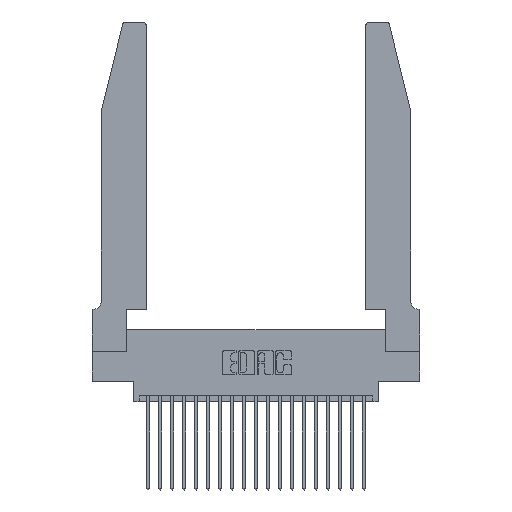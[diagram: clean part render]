
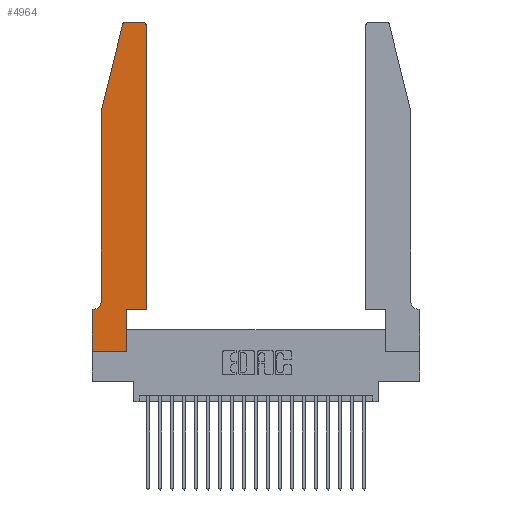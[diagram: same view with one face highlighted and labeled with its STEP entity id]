
A CAD part, top view. The second image highlights one B-rep face of the part: STEP entity #4964.
In plain terms, the highlighted planar face has unit normal (0, 0, 1).
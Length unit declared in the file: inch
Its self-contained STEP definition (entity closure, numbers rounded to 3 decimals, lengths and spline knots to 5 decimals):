
#15 = CARTESIAN_POINT ( 'NONE',  ( 0.0755, 2., 0.37 ) ) ;
#16 = LINE ( 'NONE', #1886, #22453 ) ;
#142 = CARTESIAN_POINT ( 'NONE',  ( 0.0755, 0.35, 0.37 ) ) ;
#749 = CARTESIAN_POINT ( 'NONE',  ( 0.0755, 2., 0.37 ) ) ;
#805 = DIRECTION ( 'NONE',  ( -0.239, -0.971, 0. ) ) ;
#913 = DIRECTION ( 'NONE',  ( 0., 0., 1. ) ) ;
#1130 = ORIENTED_EDGE ( 'NONE', *, *, #19484, .T. ) ;
#1185 = LINE ( 'NONE', #142, #15049 ) ;
#1429 = CIRCLE ( 'NONE', #18222, 0.03 ) ;
#1514 = EDGE_CURVE ( 'NONE', #3039, #11569, #1185, .T. ) ;
#1631 = DIRECTION ( 'NONE',  ( -1., 0., 0. ) ) ;
#1669 = DIRECTION ( 'NONE',  ( 1., 0., 0. ) ) ;
#1886 = CARTESIAN_POINT ( 'NONE',  ( 0.0755, 2., 0.37 ) ) ;
#1987 = ORIENTED_EDGE ( 'NONE', *, *, #20391, .T. ) ;
#2448 = LINE ( 'NONE', #13657, #20600 ) ;
#2665 = EDGE_CURVE ( 'NONE', #15918, #18695, #1429, .T. ) ;
#2792 = CARTESIAN_POINT ( 'NONE',  ( 0., 0.35, 0.37 ) ) ;
#3039 = VERTEX_POINT ( 'NONE', #20279 ) ;
#3133 = CARTESIAN_POINT ( 'NONE',  ( 0.0755, 0.42, 0.37 ) ) ;
#3229 = DIRECTION ( 'NONE',  ( 0., 0., -1. ) ) ;
#3417 = EDGE_CURVE ( 'NONE', #7662, #13350, #17607, .T. ) ;
#3521 = DIRECTION ( 'NONE',  ( 0., -1., 0. ) ) ;
#3588 = VERTEX_POINT ( 'NONE', #3133 ) ;
#3893 = VERTEX_POINT ( 'NONE', #21224 ) ;
#4565 = CARTESIAN_POINT ( 'NONE',  ( 0.4505, 0.35, 0.37 ) ) ;
#4650 = LINE ( 'NONE', #4565, #8903 ) ;
#4863 = AXIS2_PLACEMENT_3D ( 'NONE', #11895, #913, #13646 ) ;
#4964 = ADVANCED_FACE ( 'NONE', ( #22354 ), #22697, .T. ) ;
#5073 = LINE ( 'NONE', #21068, #18536 ) ;
#5251 = ORIENTED_EDGE ( 'NONE', *, *, #2665, .T. ) ;
#5435 = EDGE_CURVE ( 'NONE', #3588, #3039, #22332, .T. ) ;
#6041 = VERTEX_POINT ( 'NONE', #17377 ) ;
#7079 = ORIENTED_EDGE ( 'NONE', *, *, #11845, .T. ) ;
#7588 = VECTOR ( 'NONE', #21222, 39.37008 ) ;
#7662 = VERTEX_POINT ( 'NONE', #21555 ) ;
#7729 = ORIENTED_EDGE ( 'NONE', *, *, #5435, .T. ) ;
#8202 = VECTOR ( 'NONE', #3521, 39.37008 ) ;
#8570 = EDGE_CURVE ( 'NONE', #19285, #3893, #5073, .T. ) ;
#8903 = VECTOR ( 'NONE', #18604, 39.37008 ) ;
#9002 = CARTESIAN_POINT ( 'NONE',  ( 0., 0.35, 0.37 ) ) ;
#9226 = CARTESIAN_POINT ( 'NONE',  ( 0.2605, 2.75, 0.37 ) ) ;
#9789 = DIRECTION ( 'NONE',  ( 1., 0., 0. ) ) ;
#10373 = CARTESIAN_POINT ( 'NONE',  ( 0., 0., 0.37 ) ) ;
#11133 = CARTESIAN_POINT ( 'NONE',  ( 0.4505, 2.72, 0.37 ) ) ;
#11254 = EDGE_CURVE ( 'NONE', #13350, #3588, #16, .T. ) ;
#11338 = AXIS2_PLACEMENT_3D ( 'NONE', #13990, #3229, #15697 ) ;
#11569 = VERTEX_POINT ( 'NONE', #2792 ) ;
#11584 = CARTESIAN_POINT ( 'NONE',  ( 0., 0., 0.37 ) ) ;
#11598 = EDGE_CURVE ( 'NONE', #6041, #19285, #2448, .T. ) ;
#11786 = AXIS2_PLACEMENT_3D ( 'NONE', #9002, #12572, #1669 ) ;
#11804 = LINE ( 'NONE', #11584, #20334 ) ;
#11845 = EDGE_CURVE ( 'NONE', #11569, #17489, #20847, .T. ) ;
#11895 = CARTESIAN_POINT ( 'NONE',  ( 0.284, 2.72, 0.37 ) ) ;
#12526 = ORIENTED_EDGE ( 'NONE', *, *, #3417, .T. ) ;
#12572 = DIRECTION ( 'NONE',  ( 0., 0., 1. ) ) ;
#12629 = DIRECTION ( 'NONE',  ( 1., 0., 0. ) ) ;
#12766 = DIRECTION ( 'NONE',  ( 0., -1., 0. ) ) ;
#13350 = VERTEX_POINT ( 'NONE', #15 ) ;
#13523 = ORIENTED_EDGE ( 'NONE', *, *, #11598, .T. ) ;
#13646 = DIRECTION ( 'NONE',  ( 1., 0., 0. ) ) ;
#13657 = CARTESIAN_POINT ( 'NONE',  ( 0.2865, 0.35, 0.37 ) ) ;
#13990 = CARTESIAN_POINT ( 'NONE',  ( 0.0055, 0.42, 0.37 ) ) ;
#14261 = CARTESIAN_POINT ( 'NONE',  ( 0., 0., 0.37 ) ) ;
#14595 = ORIENTED_EDGE ( 'NONE', *, *, #15482, .T. ) ;
#15049 = VECTOR ( 'NONE', #1631, 39.37008 ) ;
#15482 = EDGE_CURVE ( 'NONE', #3893, #15918, #4650, .T. ) ;
#15697 = DIRECTION ( 'NONE',  ( -1., 0., 0. ) ) ;
#15918 = VERTEX_POINT ( 'NONE', #11133 ) ;
#16129 = ORIENTED_EDGE ( 'NONE', *, *, #16757, .T. ) ;
#16501 = EDGE_LOOP ( 'NONE', ( #1987, #16129, #12526, #22367, #7729, #19598, #7079, #1130, #13523, #19931, #14595, #5251 ) ) ;
#16757 = EDGE_CURVE ( 'NONE', #22017, #7662, #20162, .T. ) ;
#17085 = DIRECTION ( 'NONE',  ( 0., 1., 0. ) ) ;
#17116 = CARTESIAN_POINT ( 'NONE',  ( 0.284, 2.75, 0.37 ) ) ;
#17377 = CARTESIAN_POINT ( 'NONE',  ( 0.2865, 0., 0.37 ) ) ;
#17489 = VERTEX_POINT ( 'NONE', #10373 ) ;
#17607 = LINE ( 'NONE', #749, #20490 ) ;
#18222 = AXIS2_PLACEMENT_3D ( 'NONE', #19578, #19600, #19660 ) ;
#18536 = VECTOR ( 'NONE', #12629, 39.37008 ) ;
#18604 = DIRECTION ( 'NONE',  ( 0., 1., 0. ) ) ;
#18695 = VERTEX_POINT ( 'NONE', #19690 ) ;
#19285 = VERTEX_POINT ( 'NONE', #21260 ) ;
#19484 = EDGE_CURVE ( 'NONE', #17489, #6041, #11804, .T. ) ;
#19578 = CARTESIAN_POINT ( 'NONE',  ( 0.4205, 2.72, 0.37 ) ) ;
#19598 = ORIENTED_EDGE ( 'NONE', *, *, #1514, .T. ) ;
#19600 = DIRECTION ( 'NONE',  ( 0., 0., 1. ) ) ;
#19660 = DIRECTION ( 'NONE',  ( 1., 0., 0. ) ) ;
#19690 = CARTESIAN_POINT ( 'NONE',  ( 0.4205, 2.75, 0.37 ) ) ;
#19931 = ORIENTED_EDGE ( 'NONE', *, *, #8570, .T. ) ;
#20162 = CIRCLE ( 'NONE', #4863, 0.03 ) ;
#20279 = CARTESIAN_POINT ( 'NONE',  ( 0.0055, 0.35, 0.37 ) ) ;
#20334 = VECTOR ( 'NONE', #9789, 39.37008 ) ;
#20391 = EDGE_CURVE ( 'NONE', #18695, #22017, #20809, .T. ) ;
#20490 = VECTOR ( 'NONE', #805, 39.37008 ) ;
#20600 = VECTOR ( 'NONE', #17085, 39.37008 ) ;
#20809 = LINE ( 'NONE', #9226, #7588 ) ;
#20847 = LINE ( 'NONE', #14261, #8202 ) ;
#21068 = CARTESIAN_POINT ( 'NONE',  ( 0.4505, 0.35, 0.37 ) ) ;
#21222 = DIRECTION ( 'NONE',  ( -1., 0., 0. ) ) ;
#21224 = CARTESIAN_POINT ( 'NONE',  ( 0.4505, 0.35, 0.37 ) ) ;
#21260 = CARTESIAN_POINT ( 'NONE',  ( 0.2865, 0.35, 0.37 ) ) ;
#21555 = CARTESIAN_POINT ( 'NONE',  ( 0.25487, 2.72718, 0.37 ) ) ;
#22017 = VERTEX_POINT ( 'NONE', #17116 ) ;
#22332 = CIRCLE ( 'NONE', #11338, 0.07 ) ;
#22354 = FACE_OUTER_BOUND ( 'NONE', #16501, .T. ) ;
#22367 = ORIENTED_EDGE ( 'NONE', *, *, #11254, .T. ) ;
#22453 = VECTOR ( 'NONE', #12766, 39.37008 ) ;
#22697 = PLANE ( 'NONE',  #11786 ) ;
